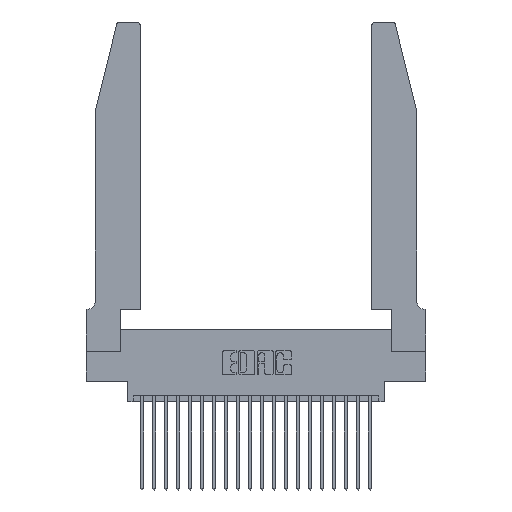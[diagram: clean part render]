
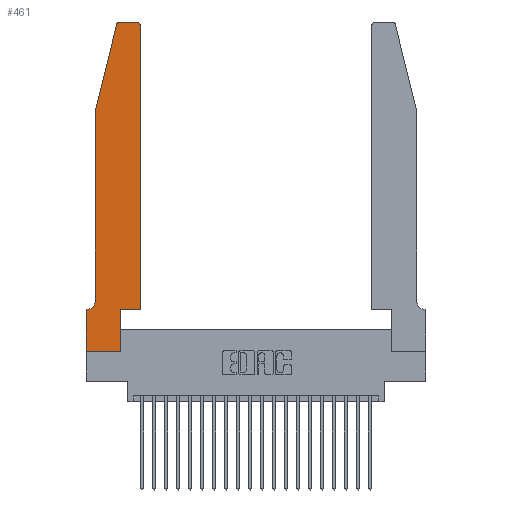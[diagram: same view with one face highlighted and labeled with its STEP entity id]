
A CAD part, top view. The second image highlights one B-rep face of the part: STEP entity #461.
In plain terms, the highlighted planar face has unit normal (0, 0, 1).
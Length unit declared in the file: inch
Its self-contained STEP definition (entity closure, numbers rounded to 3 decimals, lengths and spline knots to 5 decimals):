
#379 = VERTEX_POINT ( 'NONE', #405 ) ;
#405 = CARTESIAN_POINT ( 'NONE',  ( 0.0055, 0.35, 0.37 ) ) ;
#428 = DIRECTION ( 'NONE',  ( -1., 0., 0. ) ) ;
#461 = ADVANCED_FACE ( 'NONE', ( #12621 ), #22483, .T. ) ;
#544 = CARTESIAN_POINT ( 'NONE',  ( 0.0755, 2., 0.37 ) ) ;
#724 = CARTESIAN_POINT ( 'NONE',  ( 0.2865, 0.35, 0.37 ) ) ;
#767 = VERTEX_POINT ( 'NONE', #10463 ) ;
#1037 = CARTESIAN_POINT ( 'NONE',  ( 0.25487, 2.72718, 0.37 ) ) ;
#1378 = DIRECTION ( 'NONE',  ( 1., 0., 0. ) ) ;
#1886 = DIRECTION ( 'NONE',  ( 1., 0., 0. ) ) ;
#1908 = VECTOR ( 'NONE', #8017, 39.37008 ) ;
#2568 = DIRECTION ( 'NONE',  ( 0., 1., 0. ) ) ;
#2886 = CARTESIAN_POINT ( 'NONE',  ( 0.0055, 0.42, 0.37 ) ) ;
#3286 = CARTESIAN_POINT ( 'NONE',  ( 0.284, 2.72, 0.37 ) ) ;
#3460 = CARTESIAN_POINT ( 'NONE',  ( 0.4505, 0.35, 0.37 ) ) ;
#3899 = AXIS2_PLACEMENT_3D ( 'NONE', #5168, #17927, #7060 ) ;
#4224 = VERTEX_POINT ( 'NONE', #6224 ) ;
#4482 = CARTESIAN_POINT ( 'NONE',  ( 0.2865, 0.35, 0.37 ) ) ;
#4788 = DIRECTION ( 'NONE',  ( -1., 0., 0. ) ) ;
#4886 = CARTESIAN_POINT ( 'NONE',  ( 0.2605, 2.75, 0.37 ) ) ;
#5167 = DIRECTION ( 'NONE',  ( 1., 0., 0. ) ) ;
#5168 = CARTESIAN_POINT ( 'NONE',  ( 0.4205, 2.72, 0.37 ) ) ;
#5560 = ORIENTED_EDGE ( 'NONE', *, *, #13516, .T. ) ;
#6160 = ORIENTED_EDGE ( 'NONE', *, *, #6291, .T. ) ;
#6224 = CARTESIAN_POINT ( 'NONE',  ( 0.0755, 0.42, 0.37 ) ) ;
#6291 = EDGE_CURVE ( 'NONE', #13069, #13421, #7319, .T. ) ;
#6750 = ORIENTED_EDGE ( 'NONE', *, *, #9792, .T. ) ;
#6850 = CARTESIAN_POINT ( 'NONE',  ( 0., 0.35, 0.37 ) ) ;
#6957 = VECTOR ( 'NONE', #2568, 39.37008 ) ;
#7060 = DIRECTION ( 'NONE',  ( 1., 0., 0. ) ) ;
#7098 = CIRCLE ( 'NONE', #23494, 0.03 ) ;
#7310 = VECTOR ( 'NONE', #15913, 39.37008 ) ;
#7319 = LINE ( 'NONE', #23172, #8502 ) ;
#7332 = LINE ( 'NONE', #14587, #16419 ) ;
#7377 = CARTESIAN_POINT ( 'NONE',  ( 0.0755, 2., 0.37 ) ) ;
#7528 = VECTOR ( 'NONE', #16430, 39.37008 ) ;
#7534 = LINE ( 'NONE', #724, #6957 ) ;
#7599 = ORIENTED_EDGE ( 'NONE', *, *, #18364, .T. ) ;
#7702 = LINE ( 'NONE', #22236, #12582 ) ;
#7940 = EDGE_CURVE ( 'NONE', #9465, #4224, #21903, .T. ) ;
#8017 = DIRECTION ( 'NONE',  ( 0., -1., 0. ) ) ;
#8199 = ORIENTED_EDGE ( 'NONE', *, *, #9683, .T. ) ;
#8497 = LINE ( 'NONE', #4886, #7310 ) ;
#8502 = VECTOR ( 'NONE', #1378, 39.37008 ) ;
#8618 = DIRECTION ( 'NONE',  ( -0.239, -0.971, 0. ) ) ;
#9092 = CIRCLE ( 'NONE', #10335, 0.07 ) ;
#9465 = VERTEX_POINT ( 'NONE', #544 ) ;
#9683 = EDGE_CURVE ( 'NONE', #13195, #9465, #16257, .T. ) ;
#9758 = CIRCLE ( 'NONE', #3899, 0.03 ) ;
#9792 = EDGE_CURVE ( 'NONE', #23559, #15566, #9758, .T. ) ;
#10299 = CARTESIAN_POINT ( 'NONE',  ( 0.0755, 2., 0.37 ) ) ;
#10335 = AXIS2_PLACEMENT_3D ( 'NONE', #2886, #15752, #4788 ) ;
#10463 = CARTESIAN_POINT ( 'NONE',  ( 0.284, 2.75, 0.37 ) ) ;
#11006 = VERTEX_POINT ( 'NONE', #21159 ) ;
#11494 = VECTOR ( 'NONE', #8618, 39.37008 ) ;
#11813 = EDGE_CURVE ( 'NONE', #767, #13195, #7098, .T. ) ;
#12582 = VECTOR ( 'NONE', #428, 39.37008 ) ;
#12621 = FACE_OUTER_BOUND ( 'NONE', #17968, .T. ) ;
#13062 = EDGE_CURVE ( 'NONE', #21084, #13069, #7534, .T. ) ;
#13069 = VERTEX_POINT ( 'NONE', #4482 ) ;
#13195 = VERTEX_POINT ( 'NONE', #1037 ) ;
#13421 = VERTEX_POINT ( 'NONE', #3460 ) ;
#13516 = EDGE_CURVE ( 'NONE', #15120, #21084, #17735, .T. ) ;
#13615 = ORIENTED_EDGE ( 'NONE', *, *, #21816, .T. ) ;
#14485 = CARTESIAN_POINT ( 'NONE',  ( 0., 0., 0.37 ) ) ;
#14587 = CARTESIAN_POINT ( 'NONE',  ( 0.4505, 0.35, 0.37 ) ) ;
#15120 = VERTEX_POINT ( 'NONE', #14485 ) ;
#15566 = VERTEX_POINT ( 'NONE', #19431 ) ;
#15733 = EDGE_CURVE ( 'NONE', #379, #11006, #7702, .T. ) ;
#15752 = DIRECTION ( 'NONE',  ( 0., 0., -1. ) ) ;
#15913 = DIRECTION ( 'NONE',  ( -1., 0., 0. ) ) ;
#16112 = DIRECTION ( 'NONE',  ( 0., 0., 1. ) ) ;
#16257 = LINE ( 'NONE', #10299, #11494 ) ;
#16419 = VECTOR ( 'NONE', #21673, 39.37008 ) ;
#16430 = DIRECTION ( 'NONE',  ( 0., -1., 0. ) ) ;
#16580 = LINE ( 'NONE', #20651, #1908 ) ;
#17175 = VECTOR ( 'NONE', #1886, 39.37008 ) ;
#17439 = CARTESIAN_POINT ( 'NONE',  ( 0.2865, 0., 0.37 ) ) ;
#17628 = CARTESIAN_POINT ( 'NONE',  ( 0.4505, 2.72, 0.37 ) ) ;
#17735 = LINE ( 'NONE', #20134, #17175 ) ;
#17816 = ORIENTED_EDGE ( 'NONE', *, *, #7940, .T. ) ;
#17927 = DIRECTION ( 'NONE',  ( 0., 0., 1. ) ) ;
#17968 = EDGE_LOOP ( 'NONE', ( #7599, #21971, #8199, #17816, #13615, #23095, #19522, #5560, #20071, #6160, #20633, #6750 ) ) ;
#18364 = EDGE_CURVE ( 'NONE', #15566, #767, #8497, .T. ) ;
#18750 = AXIS2_PLACEMENT_3D ( 'NONE', #6850, #23345, #21379 ) ;
#19243 = EDGE_CURVE ( 'NONE', #11006, #15120, #16580, .T. ) ;
#19431 = CARTESIAN_POINT ( 'NONE',  ( 0.4205, 2.75, 0.37 ) ) ;
#19522 = ORIENTED_EDGE ( 'NONE', *, *, #19243, .T. ) ;
#20071 = ORIENTED_EDGE ( 'NONE', *, *, #13062, .T. ) ;
#20134 = CARTESIAN_POINT ( 'NONE',  ( 0., 0., 0.37 ) ) ;
#20633 = ORIENTED_EDGE ( 'NONE', *, *, #23079, .T. ) ;
#20651 = CARTESIAN_POINT ( 'NONE',  ( 0., 0., 0.37 ) ) ;
#21084 = VERTEX_POINT ( 'NONE', #17439 ) ;
#21159 = CARTESIAN_POINT ( 'NONE',  ( 0., 0.35, 0.37 ) ) ;
#21379 = DIRECTION ( 'NONE',  ( 1., 0., 0. ) ) ;
#21673 = DIRECTION ( 'NONE',  ( 0., 1., 0. ) ) ;
#21816 = EDGE_CURVE ( 'NONE', #4224, #379, #9092, .T. ) ;
#21903 = LINE ( 'NONE', #7377, #7528 ) ;
#21971 = ORIENTED_EDGE ( 'NONE', *, *, #11813, .T. ) ;
#22236 = CARTESIAN_POINT ( 'NONE',  ( 0.0755, 0.35, 0.37 ) ) ;
#22483 = PLANE ( 'NONE',  #18750 ) ;
#23079 = EDGE_CURVE ( 'NONE', #13421, #23559, #7332, .T. ) ;
#23095 = ORIENTED_EDGE ( 'NONE', *, *, #15733, .T. ) ;
#23172 = CARTESIAN_POINT ( 'NONE',  ( 0.4505, 0.35, 0.37 ) ) ;
#23345 = DIRECTION ( 'NONE',  ( 0., 0., 1. ) ) ;
#23494 = AXIS2_PLACEMENT_3D ( 'NONE', #3286, #16112, #5167 ) ;
#23559 = VERTEX_POINT ( 'NONE', #17628 ) ;
